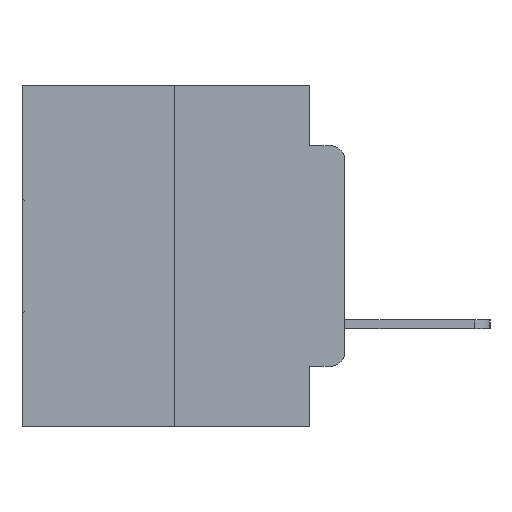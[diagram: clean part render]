
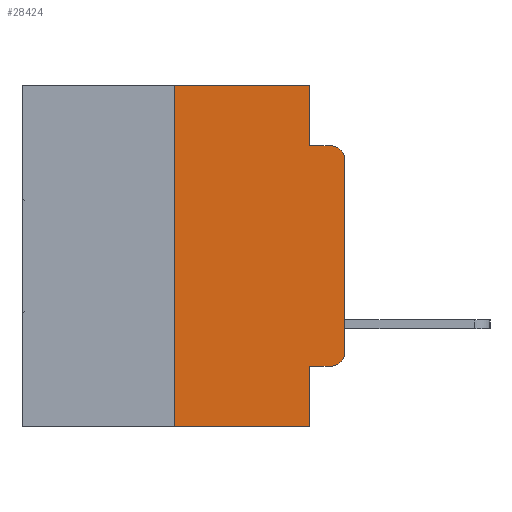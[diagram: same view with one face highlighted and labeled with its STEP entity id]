
A CAD part, left-side view. The second image highlights one B-rep face of the part: STEP entity #28424.
In plain terms, the highlighted planar face has unit normal (-1, 0, 0).
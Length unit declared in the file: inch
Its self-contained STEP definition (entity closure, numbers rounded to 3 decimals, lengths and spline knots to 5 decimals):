
#167 = VERTEX_POINT ( 'NONE', #9340 ) ;
#687 = LINE ( 'NONE', #20914, #24423 ) ;
#1032 = CARTESIAN_POINT ( 'NONE',  ( 0., 0.473, 0. ) ) ;
#1351 = EDGE_CURVE ( 'NONE', #15782, #5438, #28628, .T. ) ;
#2001 = CARTESIAN_POINT ( 'NONE',  ( 0., 0.02, -0.3915 ) ) ;
#2096 = CARTESIAN_POINT ( 'NONE',  ( 0., 0.02, -0.0885 ) ) ;
#2599 = DIRECTION ( 'NONE',  ( 0., 0., 1. ) ) ;
#2876 = DIRECTION ( 'NONE',  ( 0., -1., 0. ) ) ;
#2932 = CARTESIAN_POINT ( 'NONE',  ( 0., 0.473, -0.5 ) ) ;
#3568 = PLANE ( 'NONE',  #19080 ) ;
#3957 = DIRECTION ( 'NONE',  ( -1., 0., 0. ) ) ;
#4012 = CIRCLE ( 'NONE', #28199, 0.02 ) ;
#4519 = DIRECTION ( 'NONE',  ( 0., 0., -1. ) ) ;
#4523 = VERTEX_POINT ( 'NONE', #12729 ) ;
#4699 = CIRCLE ( 'NONE', #8448, 0.02 ) ;
#5207 = LINE ( 'NONE', #5960, #27643 ) ;
#5228 = EDGE_LOOP ( 'NONE', ( #5370, #18609, #15168, #12717, #10983, #18665, #22787, #19094, #11444, #21502 ) ) ;
#5370 = ORIENTED_EDGE ( 'NONE', *, *, #18537, .T. ) ;
#5400 = CARTESIAN_POINT ( 'NONE',  ( 0., 0.051, -0.4115 ) ) ;
#5438 = VERTEX_POINT ( 'NONE', #12029 ) ;
#5464 = DIRECTION ( 'NONE',  ( 0., -1., 0. ) ) ;
#5486 = EDGE_CURVE ( 'NONE', #19207, #26976, #25057, .T. ) ;
#5960 = CARTESIAN_POINT ( 'NONE',  ( 0., 0., 0. ) ) ;
#7540 = DIRECTION ( 'NONE',  ( 0., 0., -1. ) ) ;
#8058 = EDGE_CURVE ( 'NONE', #15782, #21613, #687, .T. ) ;
#8448 = AXIS2_PLACEMENT_3D ( 'NONE', #17773, #3957, #19985 ) ;
#8975 = LINE ( 'NONE', #18625, #14229 ) ;
#9301 = VERTEX_POINT ( 'NONE', #15844 ) ;
#9340 = CARTESIAN_POINT ( 'NONE',  ( 0., 0., -0.3915 ) ) ;
#9578 = EDGE_CURVE ( 'NONE', #9301, #19207, #11292, .T. ) ;
#10577 = VECTOR ( 'NONE', #2599, 39.37008 ) ;
#10983 = ORIENTED_EDGE ( 'NONE', *, *, #5486, .F. ) ;
#11095 = EDGE_CURVE ( 'NONE', #26976, #4523, #8975, .T. ) ;
#11292 = LINE ( 'NONE', #14349, #10577 ) ;
#11444 = ORIENTED_EDGE ( 'NONE', *, *, #1351, .T. ) ;
#11510 = FACE_OUTER_BOUND ( 'NONE', #5228, .T. ) ;
#12010 = DIRECTION ( 'NONE',  ( 0., 0., -1. ) ) ;
#12029 = CARTESIAN_POINT ( 'NONE',  ( 0., 0.02, -0.4115 ) ) ;
#12717 = ORIENTED_EDGE ( 'NONE', *, *, #11095, .F. ) ;
#12729 = CARTESIAN_POINT ( 'NONE',  ( 0., 0.051, -0.0885 ) ) ;
#12933 = DIRECTION ( 'NONE',  ( 0., 0., 1. ) ) ;
#13052 = DIRECTION ( 'NONE',  ( 0., 0., -1. ) ) ;
#13518 = CARTESIAN_POINT ( 'NONE',  ( 0., 0.051, 0. ) ) ;
#14229 = VECTOR ( 'NONE', #12010, 39.37008 ) ;
#14317 = CARTESIAN_POINT ( 'NONE',  ( 0., 0.051, -0.4115 ) ) ;
#14349 = CARTESIAN_POINT ( 'NONE',  ( 0., 0.25, 0. ) ) ;
#14414 = CARTESIAN_POINT ( 'NONE',  ( 0., 0., -0.1085 ) ) ;
#15168 = ORIENTED_EDGE ( 'NONE', *, *, #15596, .F. ) ;
#15280 = LINE ( 'NONE', #2932, #25572 ) ;
#15596 = EDGE_CURVE ( 'NONE', #4523, #29380, #28306, .T. ) ;
#15782 = VERTEX_POINT ( 'NONE', #14317 ) ;
#15844 = CARTESIAN_POINT ( 'NONE',  ( 0., 0.25, -0.5 ) ) ;
#17056 = EDGE_CURVE ( 'NONE', #25372, #29380, #4699, .T. ) ;
#17356 = VECTOR ( 'NONE', #18323, 39.37008 ) ;
#17689 = VECTOR ( 'NONE', #2876, 39.37008 ) ;
#17773 = CARTESIAN_POINT ( 'NONE',  ( 0., 0.02, -0.1085 ) ) ;
#18276 = DIRECTION ( 'NONE',  ( -1., 0., 0. ) ) ;
#18323 = DIRECTION ( 'NONE',  ( 0., -1., 0. ) ) ;
#18537 = EDGE_CURVE ( 'NONE', #167, #25372, #5207, .T. ) ;
#18609 = ORIENTED_EDGE ( 'NONE', *, *, #17056, .T. ) ;
#18625 = CARTESIAN_POINT ( 'NONE',  ( 0., 0.051, 0. ) ) ;
#18665 = ORIENTED_EDGE ( 'NONE', *, *, #9578, .F. ) ;
#19080 = AXIS2_PLACEMENT_3D ( 'NONE', #1032, #26238, #13052 ) ;
#19094 = ORIENTED_EDGE ( 'NONE', *, *, #8058, .F. ) ;
#19207 = VERTEX_POINT ( 'NONE', #25548 ) ;
#19901 = EDGE_CURVE ( 'NONE', #9301, #21613, #15280, .T. ) ;
#19937 = VECTOR ( 'NONE', #25430, 39.37008 ) ;
#19985 = DIRECTION ( 'NONE',  ( 0., 0., -1. ) ) ;
#20914 = CARTESIAN_POINT ( 'NONE',  ( 0., 0.051, 0. ) ) ;
#21502 = ORIENTED_EDGE ( 'NONE', *, *, #29359, .T. ) ;
#21613 = VERTEX_POINT ( 'NONE', #21615 ) ;
#21615 = CARTESIAN_POINT ( 'NONE',  ( 0., 0.051, -0.5 ) ) ;
#22787 = ORIENTED_EDGE ( 'NONE', *, *, #19901, .T. ) ;
#23305 = CARTESIAN_POINT ( 'NONE',  ( 0., 0.473, 0. ) ) ;
#24423 = VECTOR ( 'NONE', #7540, 39.37008 ) ;
#25057 = LINE ( 'NONE', #23305, #19937 ) ;
#25372 = VERTEX_POINT ( 'NONE', #14414 ) ;
#25430 = DIRECTION ( 'NONE',  ( 0., -1., 0. ) ) ;
#25548 = CARTESIAN_POINT ( 'NONE',  ( 0., 0.25, 0. ) ) ;
#25572 = VECTOR ( 'NONE', #5464, 39.37008 ) ;
#26238 = DIRECTION ( 'NONE',  ( 1., 0., 0. ) ) ;
#26976 = VERTEX_POINT ( 'NONE', #13518 ) ;
#26994 = CARTESIAN_POINT ( 'NONE',  ( 0., 0.051, -0.0885 ) ) ;
#27643 = VECTOR ( 'NONE', #12933, 39.37008 ) ;
#28199 = AXIS2_PLACEMENT_3D ( 'NONE', #2001, #18276, #4519 ) ;
#28306 = LINE ( 'NONE', #26994, #17356 ) ;
#28424 = ADVANCED_FACE ( 'NONE', ( #11510 ), #3568, .F. ) ;
#28628 = LINE ( 'NONE', #5400, #17689 ) ;
#29359 = EDGE_CURVE ( 'NONE', #5438, #167, #4012, .T. ) ;
#29380 = VERTEX_POINT ( 'NONE', #2096 ) ;
